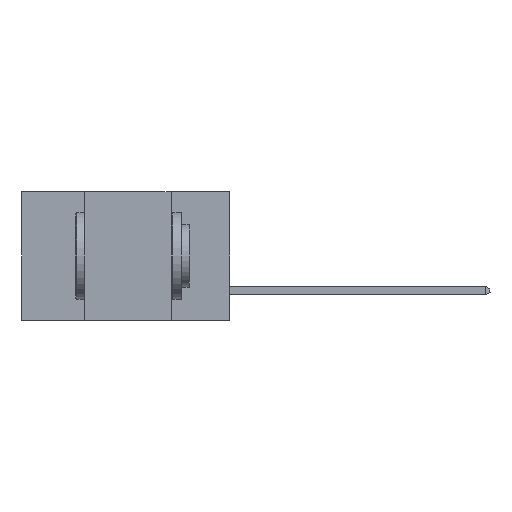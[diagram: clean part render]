
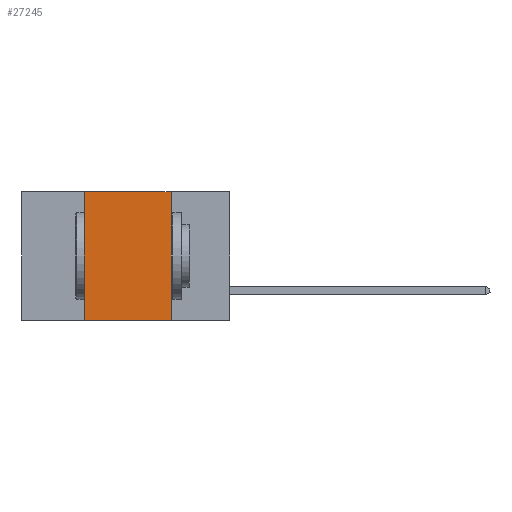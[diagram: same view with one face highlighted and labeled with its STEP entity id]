
A CAD part, left-side view. The second image highlights one B-rep face of the part: STEP entity #27245.
In plain terms, the highlighted planar face has unit normal (-1, 0, 0).
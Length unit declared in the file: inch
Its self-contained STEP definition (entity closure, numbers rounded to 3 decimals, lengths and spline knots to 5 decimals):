
#125 = PLANE ( 'NONE',  #5270 ) ;
#1098 = LINE ( 'NONE', #24464, #23129 ) ;
#2035 = DIRECTION ( 'NONE',  ( 1., 0., 0. ) ) ;
#2743 = DIRECTION ( 'NONE',  ( 0., -1., 0. ) ) ;
#3453 = ORIENTED_EDGE ( 'NONE', *, *, #10881, .T. ) ;
#3625 = CARTESIAN_POINT ( 'NONE',  ( 0., 0.42, 0. ) ) ;
#4874 = VERTEX_POINT ( 'NONE', #13942 ) ;
#5270 = AXIS2_PLACEMENT_3D ( 'NONE', #14832, #2035, #6438 ) ;
#5407 = LINE ( 'NONE', #27208, #24441 ) ;
#6438 = DIRECTION ( 'NONE',  ( 0., 0., -1. ) ) ;
#6854 = CARTESIAN_POINT ( 'NONE',  ( 0., 0.17, -0.37 ) ) ;
#7643 = CARTESIAN_POINT ( 'NONE',  ( 0., 0.42, -0.37 ) ) ;
#7936 = VERTEX_POINT ( 'NONE', #7643 ) ;
#9113 = FACE_OUTER_BOUND ( 'NONE', #23670, .T. ) ;
#10151 = DIRECTION ( 'NONE',  ( 0., 0., 1. ) ) ;
#10881 = EDGE_CURVE ( 'NONE', #7936, #13439, #20498, .T. ) ;
#11686 = DIRECTION ( 'NONE',  ( 0., -1., 0. ) ) ;
#12430 = CARTESIAN_POINT ( 'NONE',  ( 0., 0.6, -0.37 ) ) ;
#13014 = ORIENTED_EDGE ( 'NONE', *, *, #19165, .F. ) ;
#13439 = VERTEX_POINT ( 'NONE', #6854 ) ;
#13942 = CARTESIAN_POINT ( 'NONE',  ( 0., 0.42, 0. ) ) ;
#14832 = CARTESIAN_POINT ( 'NONE',  ( 0., 0.6, 0. ) ) ;
#15159 = EDGE_CURVE ( 'NONE', #7936, #4874, #17841, .T. ) ;
#16181 = VECTOR ( 'NONE', #10151, 39.37008 ) ;
#16274 = EDGE_CURVE ( 'NONE', #4874, #18175, #1098, .T. ) ;
#16608 = DIRECTION ( 'NONE',  ( 0., 0., -1. ) ) ;
#17841 = LINE ( 'NONE', #3625, #16181 ) ;
#18175 = VERTEX_POINT ( 'NONE', #19416 ) ;
#19165 = EDGE_CURVE ( 'NONE', #18175, #13439, #5407, .T. ) ;
#19416 = CARTESIAN_POINT ( 'NONE',  ( 0., 0.17, 0. ) ) ;
#20498 = LINE ( 'NONE', #12430, #21809 ) ;
#21809 = VECTOR ( 'NONE', #2743, 39.37008 ) ;
#23129 = VECTOR ( 'NONE', #11686, 39.37008 ) ;
#23158 = ORIENTED_EDGE ( 'NONE', *, *, #16274, .F. ) ;
#23670 = EDGE_LOOP ( 'NONE', ( #13014, #23158, #25014, #3453 ) ) ;
#24441 = VECTOR ( 'NONE', #16608, 39.37008 ) ;
#24464 = CARTESIAN_POINT ( 'NONE',  ( 0., 0.6, 0. ) ) ;
#25014 = ORIENTED_EDGE ( 'NONE', *, *, #15159, .F. ) ;
#27208 = CARTESIAN_POINT ( 'NONE',  ( 0., 0.17, 0. ) ) ;
#27245 = ADVANCED_FACE ( 'NONE', ( #9113 ), #125, .F. ) ;
